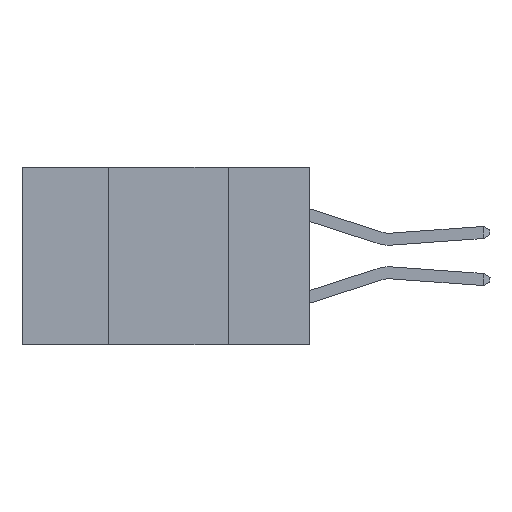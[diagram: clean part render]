
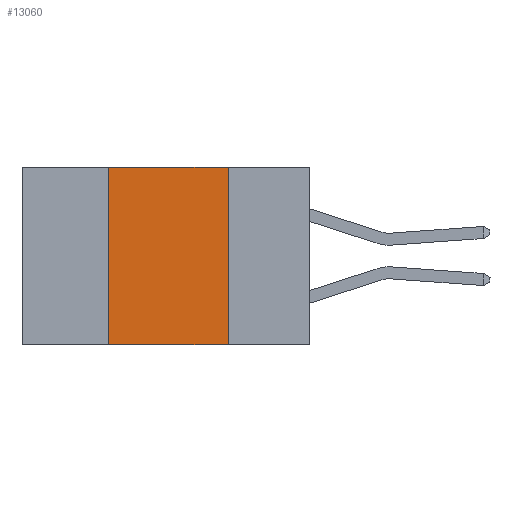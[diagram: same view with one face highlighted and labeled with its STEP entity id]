
A CAD part, left-side view. The second image highlights one B-rep face of the part: STEP entity #13060.
In plain terms, the highlighted planar face has unit normal (-1, 0, 0).
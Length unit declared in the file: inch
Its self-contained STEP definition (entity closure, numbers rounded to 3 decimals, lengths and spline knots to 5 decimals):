
#260 = VECTOR ( 'NONE', #1562, 39.37008 ) ;
#1014 = ORIENTED_EDGE ( 'NONE', *, *, #2248, .T. ) ;
#1038 = EDGE_LOOP ( 'NONE', ( #14380, #13018, #6341, #1014 ) ) ;
#1433 = VERTEX_POINT ( 'NONE', #3508 ) ;
#1562 = DIRECTION ( 'NONE',  ( 0., 0., -1. ) ) ;
#2215 = PLANE ( 'NONE',  #13273 ) ;
#2222 = EDGE_CURVE ( 'NONE', #15338, #1433, #11534, .T. ) ;
#2244 = EDGE_CURVE ( 'NONE', #17803, #16151, #7595, .T. ) ;
#2248 = EDGE_CURVE ( 'NONE', #17803, #1433, #7190, .T. ) ;
#2962 = CARTESIAN_POINT ( 'NONE',  ( 0., 0.6, 0. ) ) ;
#3449 = VECTOR ( 'NONE', #11628, 39.37008 ) ;
#3508 = CARTESIAN_POINT ( 'NONE',  ( 0., 0.17, -0.37 ) ) ;
#3766 = EDGE_CURVE ( 'NONE', #16151, #15338, #12383, .T. ) ;
#4776 = VECTOR ( 'NONE', #16812, 39.37008 ) ;
#5196 = DIRECTION ( 'NONE',  ( 0., 0., -1. ) ) ;
#6063 = CARTESIAN_POINT ( 'NONE',  ( 0., 0.17, 0. ) ) ;
#6341 = ORIENTED_EDGE ( 'NONE', *, *, #2244, .F. ) ;
#7190 = LINE ( 'NONE', #9619, #3449 ) ;
#7595 = LINE ( 'NONE', #9419, #14255 ) ;
#8673 = CARTESIAN_POINT ( 'NONE',  ( 0., 0.42, 0. ) ) ;
#9020 = CARTESIAN_POINT ( 'NONE',  ( 0., 0.42, -0.37 ) ) ;
#9419 = CARTESIAN_POINT ( 'NONE',  ( 0., 0.42, 0. ) ) ;
#9597 = CARTESIAN_POINT ( 'NONE',  ( 0., 0.17, 0. ) ) ;
#9619 = CARTESIAN_POINT ( 'NONE',  ( 0., 0.6, -0.37 ) ) ;
#11506 = DIRECTION ( 'NONE',  ( 0., 0., 1. ) ) ;
#11534 = LINE ( 'NONE', #9597, #260 ) ;
#11628 = DIRECTION ( 'NONE',  ( 0., -1., 0. ) ) ;
#11798 = FACE_OUTER_BOUND ( 'NONE', #1038, .T. ) ;
#11880 = CARTESIAN_POINT ( 'NONE',  ( 0., 0.6, 0. ) ) ;
#12383 = LINE ( 'NONE', #2962, #4776 ) ;
#13018 = ORIENTED_EDGE ( 'NONE', *, *, #3766, .F. ) ;
#13060 = ADVANCED_FACE ( 'NONE', ( #11798 ), #2215, .F. ) ;
#13234 = DIRECTION ( 'NONE',  ( 1., 0., 0. ) ) ;
#13273 = AXIS2_PLACEMENT_3D ( 'NONE', #11880, #13234, #5196 ) ;
#14255 = VECTOR ( 'NONE', #11506, 39.37008 ) ;
#14380 = ORIENTED_EDGE ( 'NONE', *, *, #2222, .F. ) ;
#15338 = VERTEX_POINT ( 'NONE', #6063 ) ;
#16151 = VERTEX_POINT ( 'NONE', #8673 ) ;
#16812 = DIRECTION ( 'NONE',  ( 0., -1., 0. ) ) ;
#17803 = VERTEX_POINT ( 'NONE', #9020 ) ;
